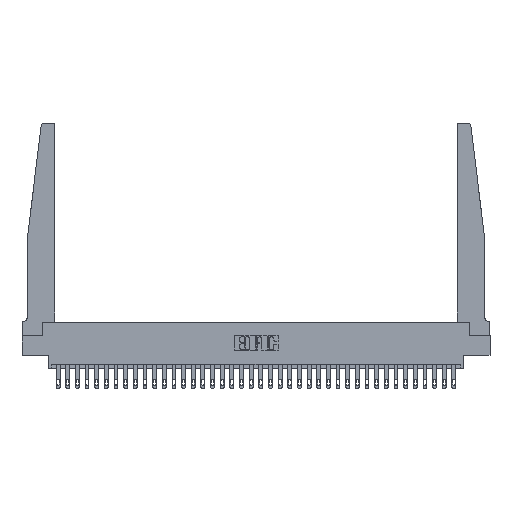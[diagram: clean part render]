
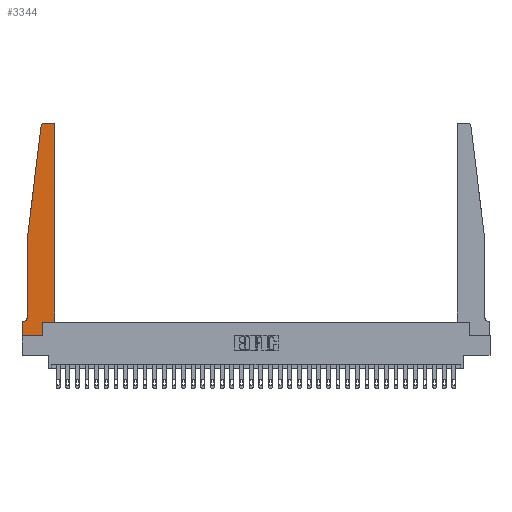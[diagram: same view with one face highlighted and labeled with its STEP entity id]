
A CAD part, top view. The second image highlights one B-rep face of the part: STEP entity #3344.
In plain terms, the highlighted planar face has unit normal (0, 0, 1).
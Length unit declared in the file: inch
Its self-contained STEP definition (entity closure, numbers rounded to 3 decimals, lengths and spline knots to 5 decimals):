
#64 = CARTESIAN_POINT ( 'NONE',  ( 0.065, 1.25, 0.37 ) ) ;
#121 = DIRECTION ( 'NONE',  ( 0., 0., -1. ) ) ;
#696 = VERTEX_POINT ( 'NONE', #6753 ) ;
#747 = DIRECTION ( 'NONE',  ( -1., 0., 0. ) ) ;
#779 = DIRECTION ( 'NONE',  ( 1., 0., 0. ) ) ;
#808 = VECTOR ( 'NONE', #16378, 39.37008 ) ;
#906 = LINE ( 'NONE', #31193, #19005 ) ;
#914 = ORIENTED_EDGE ( 'NONE', *, *, #16449, .T. ) ;
#956 = CARTESIAN_POINT ( 'NONE',  ( 0.015, 0.1875, 0.37 ) ) ;
#1193 = CARTESIAN_POINT ( 'NONE',  ( 0.065, 0.2375, 0.37 ) ) ;
#1922 = LINE ( 'NONE', #19460, #31301 ) ;
#2442 = CARTESIAN_POINT ( 'NONE',  ( 0.015, 0.2375, 0.37 ) ) ;
#2842 = DIRECTION ( 'NONE',  ( 0., -1., 0. ) ) ;
#3105 = CARTESIAN_POINT ( 'NONE',  ( 0., 0., 0.37 ) ) ;
#3330 = ORIENTED_EDGE ( 'NONE', *, *, #22172, .T. ) ;
#3344 = ADVANCED_FACE ( 'NONE', ( #24989 ), #12385, .T. ) ;
#3831 = VECTOR ( 'NONE', #17617, 39.37008 ) ;
#4325 = VERTEX_POINT ( 'NONE', #28700 ) ;
#5382 = EDGE_CURVE ( 'NONE', #696, #19610, #29617, .T. ) ;
#5774 = CIRCLE ( 'NONE', #24295, 0.03 ) ;
#5868 = VERTEX_POINT ( 'NONE', #18343 ) ;
#5895 = VERTEX_POINT ( 'NONE', #956 ) ;
#6429 = VECTOR ( 'NONE', #32499, 39.37008 ) ;
#6491 = CARTESIAN_POINT ( 'NONE',  ( 0.425, 0.18, 0.37 ) ) ;
#6492 = CARTESIAN_POINT ( 'NONE',  ( 0.2605, 0.18, 0.37 ) ) ;
#6672 = ORIENTED_EDGE ( 'NONE', *, *, #10681, .T. ) ;
#6753 = CARTESIAN_POINT ( 'NONE',  ( 0., 0.1875, 0.37 ) ) ;
#7117 = CARTESIAN_POINT ( 'NONE',  ( 0.2605, 0., 0.37 ) ) ;
#7161 = LINE ( 'NONE', #64, #6429 ) ;
#8374 = CARTESIAN_POINT ( 'NONE',  ( 0.27653, 2.75, 0.37 ) ) ;
#8739 = EDGE_CURVE ( 'NONE', #5868, #12334, #26091, .T. ) ;
#9325 = VECTOR ( 'NONE', #18722, 39.37008 ) ;
#9511 = DIRECTION ( 'NONE',  ( 1., 0., 0. ) ) ;
#9575 = CARTESIAN_POINT ( 'NONE',  ( 0., 0.1875, 0.37 ) ) ;
#9905 = DIRECTION ( 'NONE',  ( 1., 0., 0. ) ) ;
#9907 = CARTESIAN_POINT ( 'NONE',  ( 0.065, 1.25, 0.37 ) ) ;
#10355 = AXIS2_PLACEMENT_3D ( 'NONE', #2442, #121, #25457 ) ;
#10378 = CARTESIAN_POINT ( 'NONE',  ( 0., 0., 0.37 ) ) ;
#10402 = VECTOR ( 'NONE', #11590, 39.37008 ) ;
#10406 = EDGE_LOOP ( 'NONE', ( #3330, #17978, #26114, #6672, #14338, #914, #24885, #30668, #32523, #22145, #11130, #31880 ) ) ;
#10681 = EDGE_CURVE ( 'NONE', #13824, #30609, #15424, .T. ) ;
#11130 = ORIENTED_EDGE ( 'NONE', *, *, #26928, .T. ) ;
#11172 = VECTOR ( 'NONE', #779, 39.37008 ) ;
#11590 = DIRECTION ( 'NONE',  ( -1., 0., 0. ) ) ;
#11971 = DIRECTION ( 'NONE',  ( 1., 0., 0. ) ) ;
#12334 = VERTEX_POINT ( 'NONE', #20361 ) ;
#12385 = PLANE ( 'NONE',  #21360 ) ;
#13824 = VERTEX_POINT ( 'NONE', #9907 ) ;
#14338 = ORIENTED_EDGE ( 'NONE', *, *, #15359, .T. ) ;
#14464 = CARTESIAN_POINT ( 'NONE',  ( 0.395, 2.72, 0.37 ) ) ;
#15263 = CARTESIAN_POINT ( 'NONE',  ( 0.065, 1.25, 0.37 ) ) ;
#15359 = EDGE_CURVE ( 'NONE', #30609, #5895, #24661, .T. ) ;
#15424 = LINE ( 'NONE', #15263, #23647 ) ;
#15502 = VERTEX_POINT ( 'NONE', #8374 ) ;
#15849 = CARTESIAN_POINT ( 'NONE',  ( 0.27653, 2.72, 0.37 ) ) ;
#16378 = DIRECTION ( 'NONE',  ( 0., -1., 0. ) ) ;
#16418 = EDGE_CURVE ( 'NONE', #24212, #21086, #29309, .T. ) ;
#16449 = EDGE_CURVE ( 'NONE', #5895, #696, #16727, .T. ) ;
#16555 = CARTESIAN_POINT ( 'NONE',  ( 0.2605, 0.18, 0.37 ) ) ;
#16727 = LINE ( 'NONE', #31628, #10402 ) ;
#17617 = DIRECTION ( 'NONE',  ( 0., 1., 0. ) ) ;
#17978 = ORIENTED_EDGE ( 'NONE', *, *, #21736, .T. ) ;
#18160 = LINE ( 'NONE', #10378, #11172 ) ;
#18165 = AXIS2_PLACEMENT_3D ( 'NONE', #14464, #24583, #11971 ) ;
#18343 = CARTESIAN_POINT ( 'NONE',  ( 0.425, 2.72, 0.37 ) ) ;
#18722 = DIRECTION ( 'NONE',  ( 0., 1., 0. ) ) ;
#19005 = VECTOR ( 'NONE', #747, 39.37008 ) ;
#19460 = CARTESIAN_POINT ( 'NONE',  ( 0.425, 0.18, 0.37 ) ) ;
#19610 = VERTEX_POINT ( 'NONE', #3105 ) ;
#20270 = VERTEX_POINT ( 'NONE', #6491 ) ;
#20361 = CARTESIAN_POINT ( 'NONE',  ( 0.395, 2.75, 0.37 ) ) ;
#21086 = VERTEX_POINT ( 'NONE', #6492 ) ;
#21360 = AXIS2_PLACEMENT_3D ( 'NONE', #9575, #24505, #9905 ) ;
#21736 = EDGE_CURVE ( 'NONE', #15502, #4325, #5774, .T. ) ;
#22145 = ORIENTED_EDGE ( 'NONE', *, *, #26841, .T. ) ;
#22172 = EDGE_CURVE ( 'NONE', #12334, #15502, #906, .T. ) ;
#23647 = VECTOR ( 'NONE', #2842, 39.37008 ) ;
#24212 = VERTEX_POINT ( 'NONE', #7117 ) ;
#24295 = AXIS2_PLACEMENT_3D ( 'NONE', #15849, #26119, #28756 ) ;
#24505 = DIRECTION ( 'NONE',  ( 0., 0., 1. ) ) ;
#24583 = DIRECTION ( 'NONE',  ( 0., 0., 1. ) ) ;
#24661 = CIRCLE ( 'NONE', #10355, 0.05 ) ;
#24885 = ORIENTED_EDGE ( 'NONE', *, *, #5382, .T. ) ;
#24989 = FACE_OUTER_BOUND ( 'NONE', #10406, .T. ) ;
#25457 = DIRECTION ( 'NONE',  ( -1., 0., 0. ) ) ;
#26091 = CIRCLE ( 'NONE', #18165, 0.03 ) ;
#26114 = ORIENTED_EDGE ( 'NONE', *, *, #30347, .T. ) ;
#26119 = DIRECTION ( 'NONE',  ( 0., 0., 1. ) ) ;
#26719 = CARTESIAN_POINT ( 'NONE',  ( 0.425, 0.18, 0.37 ) ) ;
#26841 = EDGE_CURVE ( 'NONE', #21086, #20270, #1922, .T. ) ;
#26928 = EDGE_CURVE ( 'NONE', #20270, #5868, #27239, .T. ) ;
#27239 = LINE ( 'NONE', #26719, #3831 ) ;
#27871 = EDGE_CURVE ( 'NONE', #19610, #24212, #18160, .T. ) ;
#28700 = CARTESIAN_POINT ( 'NONE',  ( 0.24675, 2.72367, 0.37 ) ) ;
#28756 = DIRECTION ( 'NONE',  ( 1., 0., 0. ) ) ;
#28970 = CARTESIAN_POINT ( 'NONE',  ( 0., 0., 0.37 ) ) ;
#29309 = LINE ( 'NONE', #16555, #9325 ) ;
#29617 = LINE ( 'NONE', #28970, #808 ) ;
#30347 = EDGE_CURVE ( 'NONE', #4325, #13824, #7161, .T. ) ;
#30609 = VERTEX_POINT ( 'NONE', #1193 ) ;
#30668 = ORIENTED_EDGE ( 'NONE', *, *, #27871, .T. ) ;
#31193 = CARTESIAN_POINT ( 'NONE',  ( 0.25, 2.75, 0.37 ) ) ;
#31301 = VECTOR ( 'NONE', #9511, 39.37008 ) ;
#31628 = CARTESIAN_POINT ( 'NONE',  ( 0.065, 0.1875, 0.37 ) ) ;
#31880 = ORIENTED_EDGE ( 'NONE', *, *, #8739, .T. ) ;
#32499 = DIRECTION ( 'NONE',  ( -0.122, -0.992, 0. ) ) ;
#32523 = ORIENTED_EDGE ( 'NONE', *, *, #16418, .T. ) ;
